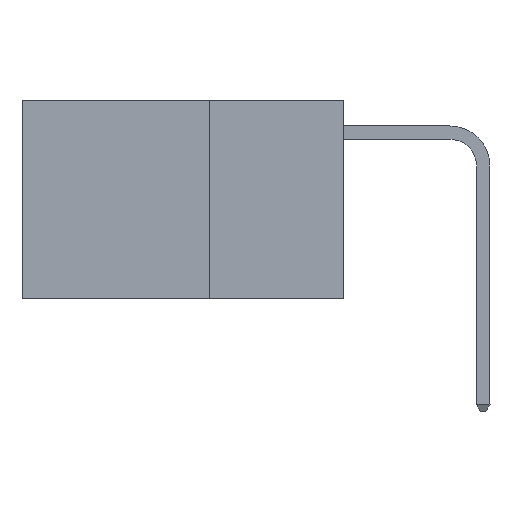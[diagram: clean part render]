
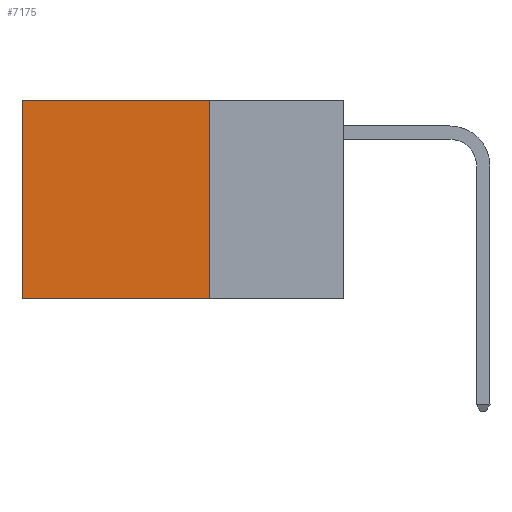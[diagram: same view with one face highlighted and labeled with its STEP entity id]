
A CAD part, left-side view. The second image highlights one B-rep face of the part: STEP entity #7175.
In plain terms, the highlighted planar face has unit normal (-1, 0, 0).
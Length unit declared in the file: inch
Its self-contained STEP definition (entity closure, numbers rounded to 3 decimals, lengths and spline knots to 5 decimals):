
#470 = EDGE_LOOP ( 'NONE', ( #14503, #7833, #4202, #7423 ) ) ;
#719 = VERTEX_POINT ( 'NONE', #4992 ) ;
#733 = CARTESIAN_POINT ( 'NONE',  ( 0.2625, 0.25, -0.37 ) ) ;
#1184 = VECTOR ( 'NONE', #3244, 39.37008 ) ;
#1803 = CARTESIAN_POINT ( 'NONE',  ( 0.2625, 0.25, 0. ) ) ;
#1988 = LINE ( 'NONE', #5919, #16057 ) ;
#2063 = VERTEX_POINT ( 'NONE', #16365 ) ;
#2468 = DIRECTION ( 'NONE',  ( 0., 0., -1. ) ) ;
#3244 = DIRECTION ( 'NONE',  ( 0., 0., -1. ) ) ;
#3830 = VECTOR ( 'NONE', #7925, 39.37008 ) ;
#4202 = ORIENTED_EDGE ( 'NONE', *, *, #15629, .F. ) ;
#4358 = VERTEX_POINT ( 'NONE', #11925 ) ;
#4992 = CARTESIAN_POINT ( 'NONE',  ( 0.2625, 0.25, 0. ) ) ;
#5016 = DIRECTION ( 'NONE',  ( 1., 0., 0. ) ) ;
#5550 = LINE ( 'NONE', #9320, #3830 ) ;
#5919 = CARTESIAN_POINT ( 'NONE',  ( 0.2625, 0.25, -0.37 ) ) ;
#6017 = EDGE_CURVE ( 'NONE', #719, #4358, #6718, .T. ) ;
#6718 = LINE ( 'NONE', #1803, #15025 ) ;
#7175 = ADVANCED_FACE ( 'NONE', ( #8949 ), #8780, .F. ) ;
#7423 = ORIENTED_EDGE ( 'NONE', *, *, #6017, .T. ) ;
#7833 = ORIENTED_EDGE ( 'NONE', *, *, #9789, .F. ) ;
#7925 = DIRECTION ( 'NONE',  ( 0., 0., -1. ) ) ;
#8780 = PLANE ( 'NONE',  #11856 ) ;
#8949 = FACE_OUTER_BOUND ( 'NONE', #470, .T. ) ;
#9320 = CARTESIAN_POINT ( 'NONE',  ( 0.2625, 0.25, 0. ) ) ;
#9789 = EDGE_CURVE ( 'NONE', #11035, #2063, #1988, .T. ) ;
#9868 = CARTESIAN_POINT ( 'NONE',  ( 0.2625, 0.25, 0. ) ) ;
#10570 = LINE ( 'NONE', #15650, #1184 ) ;
#11035 = VERTEX_POINT ( 'NONE', #733 ) ;
#11856 = AXIS2_PLACEMENT_3D ( 'NONE', #9868, #5016, #2468 ) ;
#11925 = CARTESIAN_POINT ( 'NONE',  ( 0.2625, 0.6, 0. ) ) ;
#14503 = ORIENTED_EDGE ( 'NONE', *, *, #15694, .T. ) ;
#15025 = VECTOR ( 'NONE', #15597, 39.37008 ) ;
#15597 = DIRECTION ( 'NONE',  ( 0., 1., 0. ) ) ;
#15629 = EDGE_CURVE ( 'NONE', #719, #11035, #5550, .T. ) ;
#15650 = CARTESIAN_POINT ( 'NONE',  ( 0.2625, 0.6, 0. ) ) ;
#15694 = EDGE_CURVE ( 'NONE', #4358, #2063, #10570, .T. ) ;
#16039 = DIRECTION ( 'NONE',  ( 0., 1., 0. ) ) ;
#16057 = VECTOR ( 'NONE', #16039, 39.37008 ) ;
#16365 = CARTESIAN_POINT ( 'NONE',  ( 0.2625, 0.6, -0.37 ) ) ;
